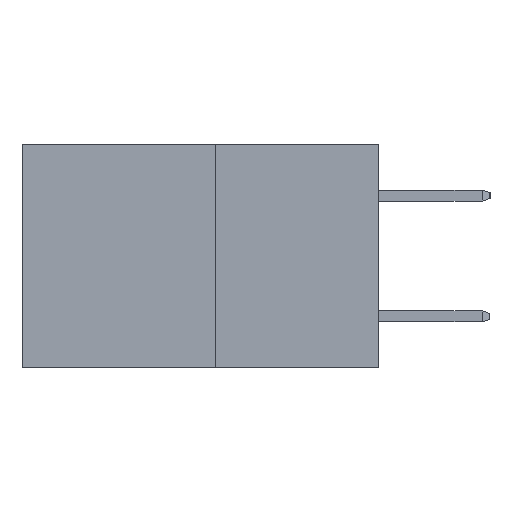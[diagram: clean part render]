
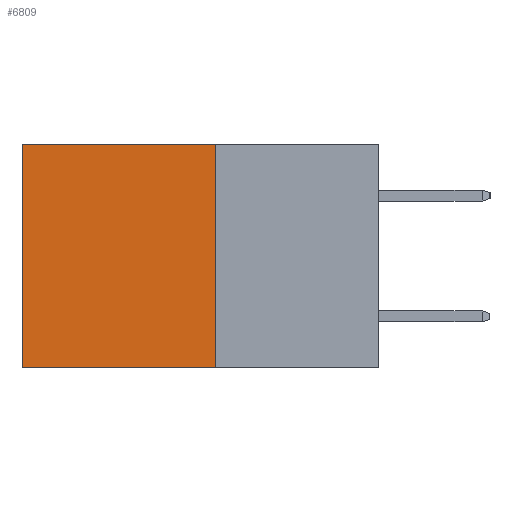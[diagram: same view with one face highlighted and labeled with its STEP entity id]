
A CAD part, left-side view. The second image highlights one B-rep face of the part: STEP entity #6809.
In plain terms, the highlighted planar face has unit normal (-1, 0, 0).
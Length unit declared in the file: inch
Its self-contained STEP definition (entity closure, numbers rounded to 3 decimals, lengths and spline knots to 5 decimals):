
#683 = PLANE ( 'NONE',  #1799 ) ;
#1116 = LINE ( 'NONE', #13580, #13298 ) ;
#1556 = LINE ( 'NONE', #13155, #13677 ) ;
#1799 = AXIS2_PLACEMENT_3D ( 'NONE', #6051, #11567, #11106 ) ;
#3027 = CARTESIAN_POINT ( 'NONE',  ( 0.277, 0.27, -0.37 ) ) ;
#3098 = ORIENTED_EDGE ( 'NONE', *, *, #14563, .F. ) ;
#3913 = DIRECTION ( 'NONE',  ( 0., 0., -1. ) ) ;
#5384 = VECTOR ( 'NONE', #8904, 39.37008 ) ;
#5388 = FACE_OUTER_BOUND ( 'NONE', #6634, .T. ) ;
#6021 = VERTEX_POINT ( 'NONE', #14006 ) ;
#6051 = CARTESIAN_POINT ( 'NONE',  ( 0.277, 0.27, -0.37 ) ) ;
#6634 = EDGE_LOOP ( 'NONE', ( #10344, #3098, #8045, #11594 ) ) ;
#6809 = ADVANCED_FACE ( 'NONE', ( #5388 ), #683, .F. ) ;
#7307 = LINE ( 'NONE', #7342, #7660 ) ;
#7342 = CARTESIAN_POINT ( 'NONE',  ( 0.277, 0.27, 0. ) ) ;
#7391 = DIRECTION ( 'NONE',  ( 0., 1., 0. ) ) ;
#7478 = VERTEX_POINT ( 'NONE', #8498 ) ;
#7660 = VECTOR ( 'NONE', #7391, 39.37008 ) ;
#8005 = EDGE_CURVE ( 'NONE', #8597, #7478, #7307, .T. ) ;
#8045 = ORIENTED_EDGE ( 'NONE', *, *, #12067, .F. ) ;
#8247 = CARTESIAN_POINT ( 'NONE',  ( 0.277, 0.59, -0.37 ) ) ;
#8498 = CARTESIAN_POINT ( 'NONE',  ( 0.277, 0.59, 0. ) ) ;
#8597 = VERTEX_POINT ( 'NONE', #15060 ) ;
#8904 = DIRECTION ( 'NONE',  ( 0., 1., 0. ) ) ;
#10229 = DIRECTION ( 'NONE',  ( 0., 0., -1. ) ) ;
#10344 = ORIENTED_EDGE ( 'NONE', *, *, #13030, .T. ) ;
#11106 = DIRECTION ( 'NONE',  ( 0., 0., -1. ) ) ;
#11567 = DIRECTION ( 'NONE',  ( 1., 0., 0. ) ) ;
#11594 = ORIENTED_EDGE ( 'NONE', *, *, #8005, .T. ) ;
#11897 = VERTEX_POINT ( 'NONE', #8247 ) ;
#11900 = LINE ( 'NONE', #3027, #5384 ) ;
#12067 = EDGE_CURVE ( 'NONE', #8597, #6021, #1556, .T. ) ;
#13030 = EDGE_CURVE ( 'NONE', #7478, #11897, #1116, .T. ) ;
#13155 = CARTESIAN_POINT ( 'NONE',  ( 0.277, 0.27, -0.37 ) ) ;
#13298 = VECTOR ( 'NONE', #10229, 39.37008 ) ;
#13580 = CARTESIAN_POINT ( 'NONE',  ( 0.277, 0.59, -0.37 ) ) ;
#13677 = VECTOR ( 'NONE', #3913, 39.37008 ) ;
#14006 = CARTESIAN_POINT ( 'NONE',  ( 0.277, 0.27, -0.37 ) ) ;
#14563 = EDGE_CURVE ( 'NONE', #6021, #11897, #11900, .T. ) ;
#15060 = CARTESIAN_POINT ( 'NONE',  ( 0.277, 0.27, 0. ) ) ;
